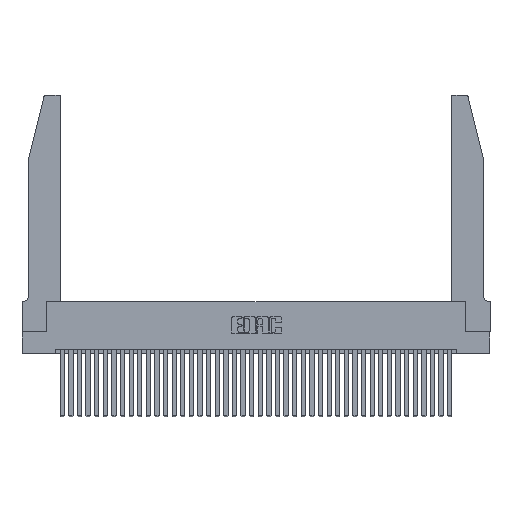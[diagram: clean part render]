
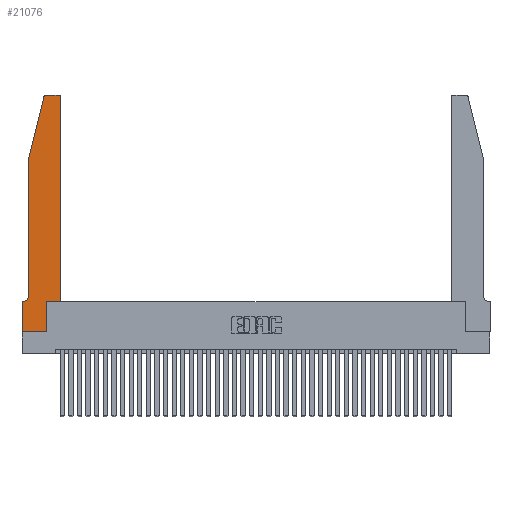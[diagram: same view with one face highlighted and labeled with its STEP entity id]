
A CAD part, top view. The second image highlights one B-rep face of the part: STEP entity #21076.
In plain terms, the highlighted planar face has unit normal (0, 0, 1).
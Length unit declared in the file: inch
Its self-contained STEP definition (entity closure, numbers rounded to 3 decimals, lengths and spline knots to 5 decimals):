
#38 = EDGE_CURVE ( 'NONE', #12025, #39953, #27993, .T. ) ;
#45 = DIRECTION ( 'NONE',  ( 1., 0., 0. ) ) ;
#272 = AXIS2_PLACEMENT_3D ( 'NONE', #30673, #37179, #45 ) ;
#829 = AXIS2_PLACEMENT_3D ( 'NONE', #32154, #20788, #14685 ) ;
#1118 = VERTEX_POINT ( 'NONE', #34859 ) ;
#1129 = VERTEX_POINT ( 'NONE', #27723 ) ;
#1302 = LINE ( 'NONE', #5193, #6153 ) ;
#1887 = LINE ( 'NONE', #27590, #11622 ) ;
#1956 = LINE ( 'NONE', #37738, #33514 ) ;
#3004 = CARTESIAN_POINT ( 'NONE',  ( 0.0755, 2., 0.37 ) ) ;
#3023 = VERTEX_POINT ( 'NONE', #4581 ) ;
#3096 = LINE ( 'NONE', #29127, #39006 ) ;
#4081 = AXIS2_PLACEMENT_3D ( 'NONE', #5996, #12688, #6124 ) ;
#4405 = VERTEX_POINT ( 'NONE', #29781 ) ;
#4509 = ORIENTED_EDGE ( 'NONE', *, *, #27888, .T. ) ;
#4581 = CARTESIAN_POINT ( 'NONE',  ( 0.0755, 0.42, 0.37 ) ) ;
#5122 = VERTEX_POINT ( 'NONE', #24780 ) ;
#5146 = CIRCLE ( 'NONE', #272, 0.03 ) ;
#5193 = CARTESIAN_POINT ( 'NONE',  ( 0.4505, 0.35, 0.37 ) ) ;
#5301 = DIRECTION ( 'NONE',  ( 1., 0., 0. ) ) ;
#5794 = VECTOR ( 'NONE', #6628, 39.37008 ) ;
#5996 = CARTESIAN_POINT ( 'NONE',  ( 0., 0.35, 0.37 ) ) ;
#6124 = DIRECTION ( 'NONE',  ( 1., 0., 0. ) ) ;
#6153 = VECTOR ( 'NONE', #35989, 39.37008 ) ;
#6628 = DIRECTION ( 'NONE',  ( -0.239, -0.971, 0. ) ) ;
#6924 = DIRECTION ( 'NONE',  ( 0., 0., -1. ) ) ;
#7348 = VECTOR ( 'NONE', #8039, 39.37008 ) ;
#7550 = DIRECTION ( 'NONE',  ( -1., 0., 0. ) ) ;
#8039 = DIRECTION ( 'NONE',  ( 0., -1., 0. ) ) ;
#8882 = ORIENTED_EDGE ( 'NONE', *, *, #32507, .T. ) ;
#9019 = DIRECTION ( 'NONE',  ( 1., 0., 0. ) ) ;
#10739 = ORIENTED_EDGE ( 'NONE', *, *, #13611, .T. ) ;
#10770 = ORIENTED_EDGE ( 'NONE', *, *, #39307, .T. ) ;
#11622 = VECTOR ( 'NONE', #9019, 39.37008 ) ;
#12019 = CARTESIAN_POINT ( 'NONE',  ( 0.25487, 2.72718, 0.37 ) ) ;
#12025 = VERTEX_POINT ( 'NONE', #31749 ) ;
#12688 = DIRECTION ( 'NONE',  ( 0., 0., 1. ) ) ;
#12813 = ORIENTED_EDGE ( 'NONE', *, *, #30777, .T. ) ;
#13358 = DIRECTION ( 'NONE',  ( 0., 1., 0. ) ) ;
#13611 = EDGE_CURVE ( 'NONE', #39953, #5122, #27565, .T. ) ;
#14685 = DIRECTION ( 'NONE',  ( 1., 0., 0. ) ) ;
#15140 = EDGE_LOOP ( 'NONE', ( #4509, #18840, #33819, #17090, #31921, #10770, #32051, #10739, #12813, #8882, #29029, #19058 ) ) ;
#17090 = ORIENTED_EDGE ( 'NONE', *, *, #18089, .T. ) ;
#17258 = LINE ( 'NONE', #29136, #31781 ) ;
#17355 = VECTOR ( 'NONE', #20977, 39.37008 ) ;
#17408 = VECTOR ( 'NONE', #5301, 39.37008 ) ;
#17839 = FACE_OUTER_BOUND ( 'NONE', #15140, .T. ) ;
#18089 = EDGE_CURVE ( 'NONE', #1118, #3023, #23860, .T. ) ;
#18840 = ORIENTED_EDGE ( 'NONE', *, *, #34047, .T. ) ;
#19058 = ORIENTED_EDGE ( 'NONE', *, *, #26794, .T. ) ;
#19418 = VERTEX_POINT ( 'NONE', #36438 ) ;
#20399 = CARTESIAN_POINT ( 'NONE',  ( 0.0755, 2., 0.37 ) ) ;
#20788 = DIRECTION ( 'NONE',  ( 0., 0., 1. ) ) ;
#20808 = EDGE_CURVE ( 'NONE', #27003, #20860, #1302, .T. ) ;
#20860 = VERTEX_POINT ( 'NONE', #29422 ) ;
#20977 = DIRECTION ( 'NONE',  ( 0., -1., 0. ) ) ;
#21024 = VERTEX_POINT ( 'NONE', #12019 ) ;
#21076 = ADVANCED_FACE ( 'NONE', ( #17839 ), #37218, .T. ) ;
#22640 = DIRECTION ( 'NONE',  ( -1., 0., 0. ) ) ;
#23860 = LINE ( 'NONE', #20399, #7348 ) ;
#24780 = CARTESIAN_POINT ( 'NONE',  ( 0.2865, 0., 0.37 ) ) ;
#25189 = LINE ( 'NONE', #3004, #5794 ) ;
#25497 = CARTESIAN_POINT ( 'NONE',  ( 0.0055, 0.42, 0.37 ) ) ;
#26794 = EDGE_CURVE ( 'NONE', #20860, #4405, #39085, .T. ) ;
#27003 = VERTEX_POINT ( 'NONE', #30524 ) ;
#27565 = LINE ( 'NONE', #34610, #17408 ) ;
#27590 = CARTESIAN_POINT ( 'NONE',  ( 0.4505, 0.35, 0.37 ) ) ;
#27723 = CARTESIAN_POINT ( 'NONE',  ( 0.2865, 0.35, 0.37 ) ) ;
#27888 = EDGE_CURVE ( 'NONE', #4405, #19418, #3096, .T. ) ;
#27993 = LINE ( 'NONE', #29612, #17355 ) ;
#28644 = DIRECTION ( 'NONE',  ( -1., 0., 0. ) ) ;
#29029 = ORIENTED_EDGE ( 'NONE', *, *, #20808, .T. ) ;
#29127 = CARTESIAN_POINT ( 'NONE',  ( 0.2605, 2.75, 0.37 ) ) ;
#29136 = CARTESIAN_POINT ( 'NONE',  ( 0.0755, 0.35, 0.37 ) ) ;
#29422 = CARTESIAN_POINT ( 'NONE',  ( 0.4505, 2.72, 0.37 ) ) ;
#29612 = CARTESIAN_POINT ( 'NONE',  ( 0., 0., 0.37 ) ) ;
#29781 = CARTESIAN_POINT ( 'NONE',  ( 0.4205, 2.75, 0.37 ) ) ;
#30524 = CARTESIAN_POINT ( 'NONE',  ( 0.4505, 0.35, 0.37 ) ) ;
#30673 = CARTESIAN_POINT ( 'NONE',  ( 0.284, 2.72, 0.37 ) ) ;
#30777 = EDGE_CURVE ( 'NONE', #5122, #1129, #1956, .T. ) ;
#31250 = CARTESIAN_POINT ( 'NONE',  ( 0., 0., 0.37 ) ) ;
#31336 = EDGE_CURVE ( 'NONE', #21024, #1118, #25189, .T. ) ;
#31749 = CARTESIAN_POINT ( 'NONE',  ( 0., 0.35, 0.37 ) ) ;
#31781 = VECTOR ( 'NONE', #22640, 39.37008 ) ;
#31921 = ORIENTED_EDGE ( 'NONE', *, *, #38697, .T. ) ;
#32051 = ORIENTED_EDGE ( 'NONE', *, *, #38, .T. ) ;
#32154 = CARTESIAN_POINT ( 'NONE',  ( 0.4205, 2.72, 0.37 ) ) ;
#32507 = EDGE_CURVE ( 'NONE', #1129, #27003, #1887, .T. ) ;
#33514 = VECTOR ( 'NONE', #13358, 39.37008 ) ;
#33819 = ORIENTED_EDGE ( 'NONE', *, *, #31336, .T. ) ;
#34047 = EDGE_CURVE ( 'NONE', #19418, #21024, #5146, .T. ) ;
#34610 = CARTESIAN_POINT ( 'NONE',  ( 0., 0., 0.37 ) ) ;
#34859 = CARTESIAN_POINT ( 'NONE',  ( 0.0755, 2., 0.37 ) ) ;
#35989 = DIRECTION ( 'NONE',  ( 0., 1., 0. ) ) ;
#36438 = CARTESIAN_POINT ( 'NONE',  ( 0.284, 2.75, 0.37 ) ) ;
#36941 = VERTEX_POINT ( 'NONE', #38676 ) ;
#37179 = DIRECTION ( 'NONE',  ( 0., 0., 1. ) ) ;
#37218 = PLANE ( 'NONE',  #4081 ) ;
#37738 = CARTESIAN_POINT ( 'NONE',  ( 0.2865, 0.35, 0.37 ) ) ;
#38075 = CIRCLE ( 'NONE', #39226, 0.07 ) ;
#38676 = CARTESIAN_POINT ( 'NONE',  ( 0.0055, 0.35, 0.37 ) ) ;
#38697 = EDGE_CURVE ( 'NONE', #3023, #36941, #38075, .T. ) ;
#39006 = VECTOR ( 'NONE', #7550, 39.37008 ) ;
#39085 = CIRCLE ( 'NONE', #829, 0.03 ) ;
#39226 = AXIS2_PLACEMENT_3D ( 'NONE', #25497, #6924, #28644 ) ;
#39307 = EDGE_CURVE ( 'NONE', #36941, #12025, #17258, .T. ) ;
#39953 = VERTEX_POINT ( 'NONE', #31250 ) ;
